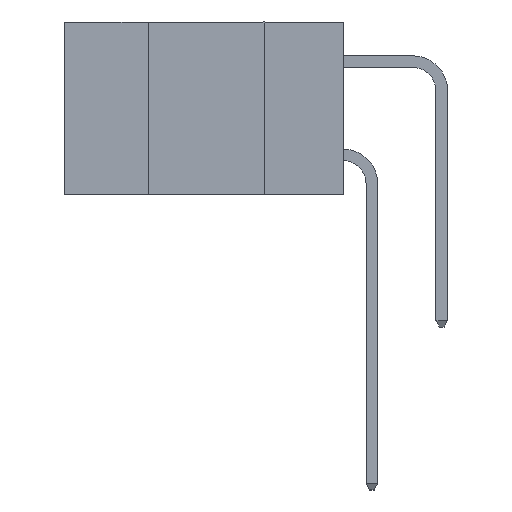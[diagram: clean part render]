
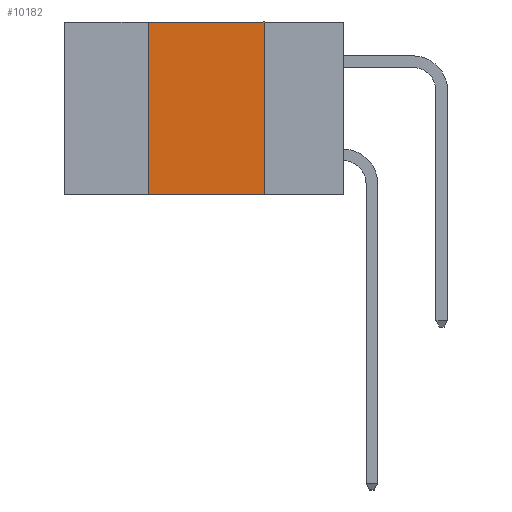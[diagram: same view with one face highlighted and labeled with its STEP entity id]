
A CAD part, left-side view. The second image highlights one B-rep face of the part: STEP entity #10182.
In plain terms, the highlighted planar face has unit normal (-1, 0, 0).
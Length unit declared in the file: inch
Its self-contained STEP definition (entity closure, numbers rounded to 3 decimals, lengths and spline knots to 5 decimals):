
#896 = CARTESIAN_POINT ( 'NONE',  ( 0., 0.17, -0.37 ) ) ;
#965 = VECTOR ( 'NONE', #11069, 39.37008 ) ;
#2440 = LINE ( 'NONE', #6325, #6628 ) ;
#2693 = LINE ( 'NONE', #4800, #4296 ) ;
#2932 = AXIS2_PLACEMENT_3D ( 'NONE', #4760, #11241, #4806 ) ;
#3442 = CARTESIAN_POINT ( 'NONE',  ( 0., 0.42, -0.37 ) ) ;
#3473 = LINE ( 'NONE', #7364, #965 ) ;
#3781 = CARTESIAN_POINT ( 'NONE',  ( 0., 0.42, 0. ) ) ;
#3830 = LINE ( 'NONE', #7546, #11770 ) ;
#3931 = ORIENTED_EDGE ( 'NONE', *, *, #7070, .F. ) ;
#4296 = VECTOR ( 'NONE', #7658, 39.37008 ) ;
#4760 = CARTESIAN_POINT ( 'NONE',  ( 0., 0.6, 0. ) ) ;
#4774 = EDGE_CURVE ( 'NONE', #9380, #9116, #3830, .T. ) ;
#4800 = CARTESIAN_POINT ( 'NONE',  ( 0., 0.6, -0.37 ) ) ;
#4806 = DIRECTION ( 'NONE',  ( 0., 0., -1. ) ) ;
#5166 = VERTEX_POINT ( 'NONE', #896 ) ;
#5942 = CARTESIAN_POINT ( 'NONE',  ( 0., 0.17, 0. ) ) ;
#6325 = CARTESIAN_POINT ( 'NONE',  ( 0., 0.17, -0.37 ) ) ;
#6628 = VECTOR ( 'NONE', #7124, 39.37008 ) ;
#6648 = ORIENTED_EDGE ( 'NONE', *, *, #8344, .T. ) ;
#7070 = EDGE_CURVE ( 'NONE', #9171, #5166, #2440, .T. ) ;
#7085 = EDGE_CURVE ( 'NONE', #9116, #9171, #3473, .T. ) ;
#7124 = DIRECTION ( 'NONE',  ( 0., 0., -1. ) ) ;
#7364 = CARTESIAN_POINT ( 'NONE',  ( 0., 0.6, 0. ) ) ;
#7546 = CARTESIAN_POINT ( 'NONE',  ( 0., 0.42, -0.37 ) ) ;
#7658 = DIRECTION ( 'NONE',  ( 0., -1., 0. ) ) ;
#8344 = EDGE_CURVE ( 'NONE', #9380, #5166, #2693, .T. ) ;
#8476 = PLANE ( 'NONE',  #2932 ) ;
#9116 = VERTEX_POINT ( 'NONE', #3781 ) ;
#9171 = VERTEX_POINT ( 'NONE', #5942 ) ;
#9376 = DIRECTION ( 'NONE',  ( 0., 0., 1. ) ) ;
#9380 = VERTEX_POINT ( 'NONE', #3442 ) ;
#10182 = ADVANCED_FACE ( 'NONE', ( #11458 ), #8476, .F. ) ;
#10818 = ORIENTED_EDGE ( 'NONE', *, *, #7085, .F. ) ;
#11069 = DIRECTION ( 'NONE',  ( 0., -1., 0. ) ) ;
#11082 = EDGE_LOOP ( 'NONE', ( #3931, #10818, #11310, #6648 ) ) ;
#11241 = DIRECTION ( 'NONE',  ( 1., 0., 0. ) ) ;
#11310 = ORIENTED_EDGE ( 'NONE', *, *, #4774, .F. ) ;
#11458 = FACE_OUTER_BOUND ( 'NONE', #11082, .T. ) ;
#11770 = VECTOR ( 'NONE', #9376, 39.37008 ) ;
